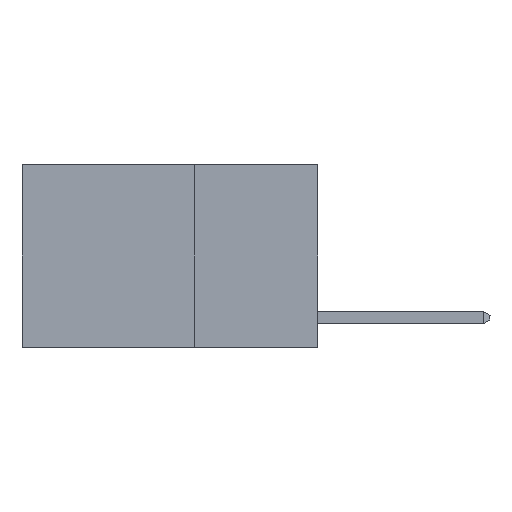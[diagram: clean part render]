
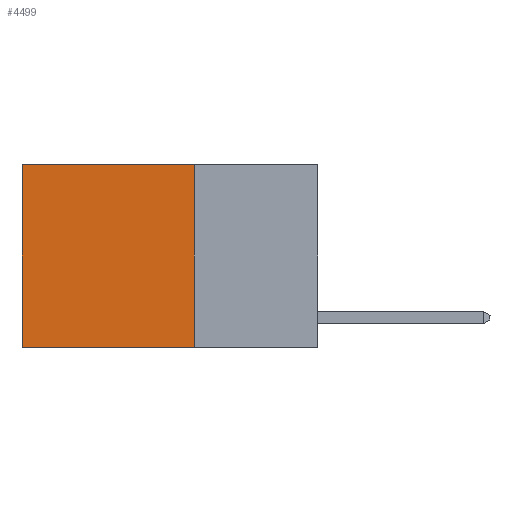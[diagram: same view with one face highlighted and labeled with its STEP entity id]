
A CAD part, left-side view. The second image highlights one B-rep face of the part: STEP entity #4499.
In plain terms, the highlighted planar face has unit normal (-1, 0, 0).
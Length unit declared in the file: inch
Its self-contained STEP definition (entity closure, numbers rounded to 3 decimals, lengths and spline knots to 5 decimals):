
#294 = CARTESIAN_POINT ( 'NONE',  ( 0.2625, 0.6, -0.37 ) ) ;
#1094 = AXIS2_PLACEMENT_3D ( 'NONE', #18310, #5255, #9730 ) ;
#2069 = CARTESIAN_POINT ( 'NONE',  ( 0.2625, 0.6, 0. ) ) ;
#2259 = LINE ( 'NONE', #18187, #18156 ) ;
#2620 = VERTEX_POINT ( 'NONE', #5680 ) ;
#3146 = VECTOR ( 'NONE', #12239, 39.37008 ) ;
#3659 = LINE ( 'NONE', #9309, #3146 ) ;
#3891 = VECTOR ( 'NONE', #13564, 39.37008 ) ;
#4499 = ADVANCED_FACE ( 'NONE', ( #15299 ), #6681, .F. ) ;
#4762 = DIRECTION ( 'NONE',  ( 0., 0., -1. ) ) ;
#5231 = ORIENTED_EDGE ( 'NONE', *, *, #16854, .T. ) ;
#5255 = DIRECTION ( 'NONE',  ( 1., 0., 0. ) ) ;
#5552 = EDGE_CURVE ( 'NONE', #6970, #2620, #5838, .T. ) ;
#5680 = CARTESIAN_POINT ( 'NONE',  ( 0.2625, 0.25, -0.37 ) ) ;
#5838 = LINE ( 'NONE', #8750, #14059 ) ;
#6246 = VERTEX_POINT ( 'NONE', #294 ) ;
#6488 = ORIENTED_EDGE ( 'NONE', *, *, #12440, .T. ) ;
#6681 = PLANE ( 'NONE',  #1094 ) ;
#6970 = VERTEX_POINT ( 'NONE', #11441 ) ;
#8750 = CARTESIAN_POINT ( 'NONE',  ( 0.2625, 0.25, 0. ) ) ;
#8951 = ORIENTED_EDGE ( 'NONE', *, *, #5552, .F. ) ;
#9308 = DIRECTION ( 'NONE',  ( 0., 1., 0. ) ) ;
#9309 = CARTESIAN_POINT ( 'NONE',  ( 0.2625, 0.25, 0. ) ) ;
#9536 = ORIENTED_EDGE ( 'NONE', *, *, #16773, .F. ) ;
#9682 = LINE ( 'NONE', #2069, #3891 ) ;
#9730 = DIRECTION ( 'NONE',  ( 0., 0., -1. ) ) ;
#11441 = CARTESIAN_POINT ( 'NONE',  ( 0.2625, 0.25, 0. ) ) ;
#12104 = CARTESIAN_POINT ( 'NONE',  ( 0.2625, 0.6, 0. ) ) ;
#12239 = DIRECTION ( 'NONE',  ( 0., 1., 0. ) ) ;
#12440 = EDGE_CURVE ( 'NONE', #6970, #12894, #3659, .T. ) ;
#12894 = VERTEX_POINT ( 'NONE', #12104 ) ;
#13264 = EDGE_LOOP ( 'NONE', ( #5231, #9536, #8951, #6488 ) ) ;
#13564 = DIRECTION ( 'NONE',  ( 0., 0., -1. ) ) ;
#14059 = VECTOR ( 'NONE', #4762, 39.37008 ) ;
#15299 = FACE_OUTER_BOUND ( 'NONE', #13264, .T. ) ;
#16773 = EDGE_CURVE ( 'NONE', #2620, #6246, #2259, .T. ) ;
#16854 = EDGE_CURVE ( 'NONE', #12894, #6246, #9682, .T. ) ;
#18156 = VECTOR ( 'NONE', #9308, 39.37008 ) ;
#18187 = CARTESIAN_POINT ( 'NONE',  ( 0.2625, 0.25, -0.37 ) ) ;
#18310 = CARTESIAN_POINT ( 'NONE',  ( 0.2625, 0.25, 0. ) ) ;
